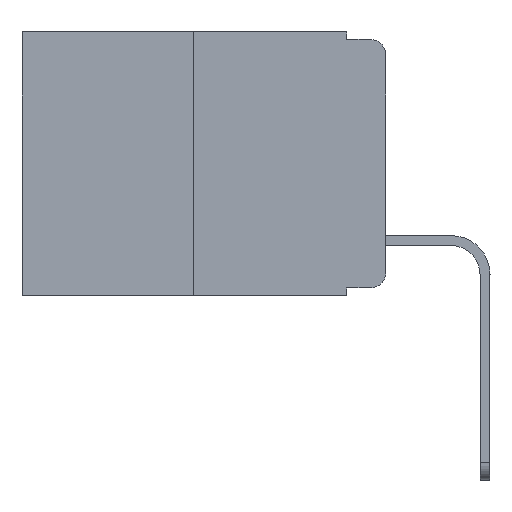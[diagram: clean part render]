
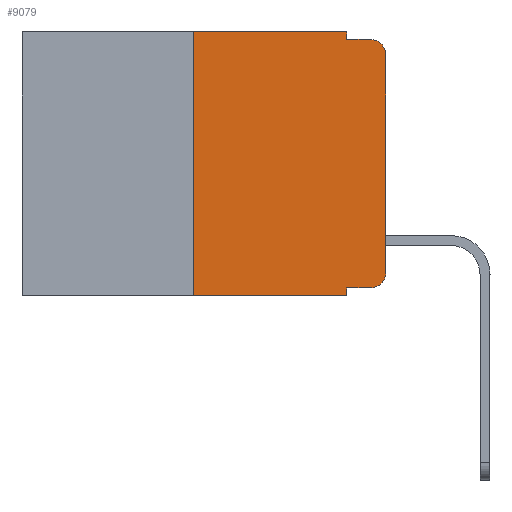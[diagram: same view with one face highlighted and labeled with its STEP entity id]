
A CAD part, left-side view. The second image highlights one B-rep face of the part: STEP entity #9079.
In plain terms, the highlighted planar face has unit normal (-1, 0, 0).
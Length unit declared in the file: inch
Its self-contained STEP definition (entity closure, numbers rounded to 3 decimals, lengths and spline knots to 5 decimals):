
#161 = EDGE_CURVE ( 'NONE', #2047, #10522, #9075, .T. ) ;
#581 = AXIS2_PLACEMENT_3D ( 'NONE', #7880, #4437, #1176 ) ;
#659 = VERTEX_POINT ( 'NONE', #6623 ) ;
#770 = ORIENTED_EDGE ( 'NONE', *, *, #14072, .T. ) ;
#823 = CARTESIAN_POINT ( 'NONE',  ( 0., 0.051, 0. ) ) ;
#1106 = CARTESIAN_POINT ( 'NONE',  ( 0., 0.051, -0.01 ) ) ;
#1171 = VECTOR ( 'NONE', #12158, 39.37008 ) ;
#1176 = DIRECTION ( 'NONE',  ( 0., 0., -1. ) ) ;
#1527 = DIRECTION ( 'NONE',  ( 0., -1., 0. ) ) ;
#1563 = VECTOR ( 'NONE', #5927, 39.37008 ) ;
#1736 = LINE ( 'NONE', #3517, #4869 ) ;
#1790 = PLANE ( 'NONE',  #12629 ) ;
#1888 = LINE ( 'NONE', #4975, #10463 ) ;
#1894 = DIRECTION ( 'NONE',  ( 0., -1., 0. ) ) ;
#2047 = VERTEX_POINT ( 'NONE', #4943 ) ;
#2103 = DIRECTION ( 'NONE',  ( 0., 0., -1. ) ) ;
#2860 = DIRECTION ( 'NONE',  ( 1., 0., 0. ) ) ;
#2994 = CIRCLE ( 'NONE', #5416, 0.02 ) ;
#3093 = VECTOR ( 'NONE', #10915, 39.37008 ) ;
#3305 = EDGE_LOOP ( 'NONE', ( #9592, #6971, #11842, #11942, #10474, #6906, #770, #10938, #13505, #12738 ) ) ;
#3502 = CARTESIAN_POINT ( 'NONE',  ( 0., 0.051, 0. ) ) ;
#3517 = CARTESIAN_POINT ( 'NONE',  ( 0., 0.473, 0. ) ) ;
#3646 = EDGE_CURVE ( 'NONE', #10522, #9061, #2994, .T. ) ;
#3809 = VERTEX_POINT ( 'NONE', #13875 ) ;
#3945 = LINE ( 'NONE', #823, #3093 ) ;
#3983 = LINE ( 'NONE', #6064, #1563 ) ;
#4389 = LINE ( 'NONE', #1106, #7017 ) ;
#4437 = DIRECTION ( 'NONE',  ( -1., 0., 0. ) ) ;
#4869 = VECTOR ( 'NONE', #1527, 39.37008 ) ;
#4943 = CARTESIAN_POINT ( 'NONE',  ( 0., 0.051, -0.333 ) ) ;
#4975 = CARTESIAN_POINT ( 'NONE',  ( 0., 0.051, 0. ) ) ;
#5030 = DIRECTION ( 'NONE',  ( 0., 0., -1. ) ) ;
#5342 = VECTOR ( 'NONE', #10568, 39.37008 ) ;
#5416 = AXIS2_PLACEMENT_3D ( 'NONE', #12358, #8841, #2103 ) ;
#5696 = CARTESIAN_POINT ( 'NONE',  ( 0., 0.051, -0.343 ) ) ;
#5927 = DIRECTION ( 'NONE',  ( 0., 0., 1. ) ) ;
#6055 = CARTESIAN_POINT ( 'NONE',  ( 0., 0., 0. ) ) ;
#6064 = CARTESIAN_POINT ( 'NONE',  ( 0., 0.25, 0. ) ) ;
#6123 = EDGE_CURVE ( 'NONE', #9562, #3809, #12922, .T. ) ;
#6345 = VERTEX_POINT ( 'NONE', #10513 ) ;
#6623 = CARTESIAN_POINT ( 'NONE',  ( 0., 0.051, -0.01 ) ) ;
#6906 = ORIENTED_EDGE ( 'NONE', *, *, #11480, .F. ) ;
#6971 = ORIENTED_EDGE ( 'NONE', *, *, #6123, .T. ) ;
#7017 = VECTOR ( 'NONE', #7663, 39.37008 ) ;
#7096 = LINE ( 'NONE', #6055, #5342 ) ;
#7203 = DIRECTION ( 'NONE',  ( 0., 0., -1. ) ) ;
#7663 = DIRECTION ( 'NONE',  ( 0., -1., 0. ) ) ;
#7880 = CARTESIAN_POINT ( 'NONE',  ( 0., 0.02, -0.03 ) ) ;
#7964 = CARTESIAN_POINT ( 'NONE',  ( 0., 0.02, -0.333 ) ) ;
#8414 = CARTESIAN_POINT ( 'NONE',  ( 0., 0.473, -0.343 ) ) ;
#8511 = EDGE_CURVE ( 'NONE', #659, #3809, #4389, .T. ) ;
#8701 = VERTEX_POINT ( 'NONE', #5696 ) ;
#8841 = DIRECTION ( 'NONE',  ( -1., 0., 0. ) ) ;
#9061 = VERTEX_POINT ( 'NONE', #11784 ) ;
#9075 = LINE ( 'NONE', #11910, #1171 ) ;
#9079 = ADVANCED_FACE ( 'NONE', ( #12820 ), #1790, .F. ) ;
#9556 = LINE ( 'NONE', #8414, #13072 ) ;
#9562 = VERTEX_POINT ( 'NONE', #12857 ) ;
#9592 = ORIENTED_EDGE ( 'NONE', *, *, #13421, .T. ) ;
#9829 = VERTEX_POINT ( 'NONE', #13205 ) ;
#10463 = VECTOR ( 'NONE', #5030, 39.37008 ) ;
#10474 = ORIENTED_EDGE ( 'NONE', *, *, #11376, .F. ) ;
#10513 = CARTESIAN_POINT ( 'NONE',  ( 0., 0.25, -0.343 ) ) ;
#10522 = VERTEX_POINT ( 'NONE', #7964 ) ;
#10568 = DIRECTION ( 'NONE',  ( 0., 0., 1. ) ) ;
#10915 = DIRECTION ( 'NONE',  ( 0., 0., -1. ) ) ;
#10938 = ORIENTED_EDGE ( 'NONE', *, *, #12951, .F. ) ;
#11376 = EDGE_CURVE ( 'NONE', #9829, #11926, #1736, .T. ) ;
#11480 = EDGE_CURVE ( 'NONE', #6345, #9829, #3983, .T. ) ;
#11784 = CARTESIAN_POINT ( 'NONE',  ( 0., 0., -0.313 ) ) ;
#11842 = ORIENTED_EDGE ( 'NONE', *, *, #8511, .F. ) ;
#11910 = CARTESIAN_POINT ( 'NONE',  ( 0., 0.051, -0.333 ) ) ;
#11926 = VERTEX_POINT ( 'NONE', #3502 ) ;
#11942 = ORIENTED_EDGE ( 'NONE', *, *, #13623, .F. ) ;
#12158 = DIRECTION ( 'NONE',  ( 0., -1., 0. ) ) ;
#12358 = CARTESIAN_POINT ( 'NONE',  ( 0., 0.02, -0.313 ) ) ;
#12629 = AXIS2_PLACEMENT_3D ( 'NONE', #12828, #2860, #7203 ) ;
#12738 = ORIENTED_EDGE ( 'NONE', *, *, #3646, .T. ) ;
#12820 = FACE_OUTER_BOUND ( 'NONE', #3305, .T. ) ;
#12828 = CARTESIAN_POINT ( 'NONE',  ( 0., 0.473, 0. ) ) ;
#12857 = CARTESIAN_POINT ( 'NONE',  ( 0., 0., -0.03 ) ) ;
#12922 = CIRCLE ( 'NONE', #581, 0.02 ) ;
#12951 = EDGE_CURVE ( 'NONE', #2047, #8701, #1888, .T. ) ;
#13072 = VECTOR ( 'NONE', #1894, 39.37008 ) ;
#13205 = CARTESIAN_POINT ( 'NONE',  ( 0., 0.25, 0. ) ) ;
#13421 = EDGE_CURVE ( 'NONE', #9061, #9562, #7096, .T. ) ;
#13505 = ORIENTED_EDGE ( 'NONE', *, *, #161, .T. ) ;
#13623 = EDGE_CURVE ( 'NONE', #11926, #659, #3945, .T. ) ;
#13875 = CARTESIAN_POINT ( 'NONE',  ( 0., 0.02, -0.01 ) ) ;
#14072 = EDGE_CURVE ( 'NONE', #6345, #8701, #9556, .T. ) ;
